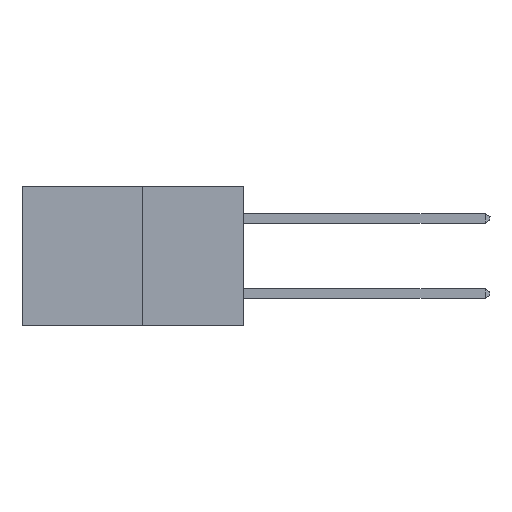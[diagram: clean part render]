
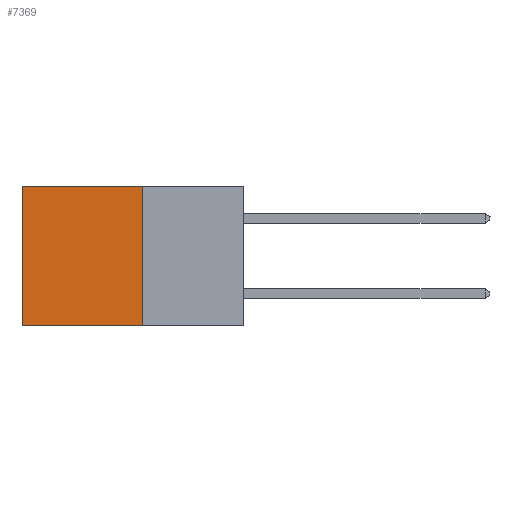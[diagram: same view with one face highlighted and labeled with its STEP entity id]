
A CAD part, left-side view. The second image highlights one B-rep face of the part: STEP entity #7369.
In plain terms, the highlighted planar face has unit normal (-1, 0, 0).
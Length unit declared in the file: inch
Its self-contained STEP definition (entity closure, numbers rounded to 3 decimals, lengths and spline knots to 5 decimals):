
#693 = AXIS2_PLACEMENT_3D ( 'NONE', #26904, #10281, #29672 ) ;
#1352 = VERTEX_POINT ( 'NONE', #14864 ) ;
#1359 = CARTESIAN_POINT ( 'NONE',  ( 0.277, 0.27, -0.37 ) ) ;
#3016 = VECTOR ( 'NONE', #18110, 39.37008 ) ;
#5978 = ORIENTED_EDGE ( 'NONE', *, *, #6654, .T. ) ;
#6654 = EDGE_CURVE ( 'NONE', #26735, #32204, #28831, .T. ) ;
#6737 = CARTESIAN_POINT ( 'NONE',  ( 0.277, 0.59, 0. ) ) ;
#6918 = ORIENTED_EDGE ( 'NONE', *, *, #29499, .F. ) ;
#7369 = ADVANCED_FACE ( 'NONE', ( #20980 ), #7477, .F. ) ;
#7477 = PLANE ( 'NONE',  #693 ) ;
#10281 = DIRECTION ( 'NONE',  ( 1., 0., 0. ) ) ;
#10402 = VECTOR ( 'NONE', #33155, 39.37008 ) ;
#11714 = EDGE_CURVE ( 'NONE', #1352, #35198, #17893, .T. ) ;
#12230 = CARTESIAN_POINT ( 'NONE',  ( 0.277, 0.59, -0.37 ) ) ;
#12426 = VECTOR ( 'NONE', #29361, 39.37008 ) ;
#12638 = DIRECTION ( 'NONE',  ( 0., 0., -1. ) ) ;
#14152 = LINE ( 'NONE', #31970, #12426 ) ;
#14864 = CARTESIAN_POINT ( 'NONE',  ( 0.277, 0.27, 0. ) ) ;
#17893 = LINE ( 'NONE', #1359, #3016 ) ;
#18110 = DIRECTION ( 'NONE',  ( 0., 0., -1. ) ) ;
#18461 = EDGE_CURVE ( 'NONE', #1352, #26735, #14152, .T. ) ;
#20570 = ORIENTED_EDGE ( 'NONE', *, *, #11714, .F. ) ;
#20980 = FACE_OUTER_BOUND ( 'NONE', #26748, .T. ) ;
#21452 = VECTOR ( 'NONE', #12638, 39.37008 ) ;
#26456 = CARTESIAN_POINT ( 'NONE',  ( 0.277, 0.59, -0.37 ) ) ;
#26735 = VERTEX_POINT ( 'NONE', #6737 ) ;
#26748 = EDGE_LOOP ( 'NONE', ( #5978, #6918, #20570, #31355 ) ) ;
#26904 = CARTESIAN_POINT ( 'NONE',  ( 0.277, 0.27, -0.37 ) ) ;
#28831 = LINE ( 'NONE', #26456, #21452 ) ;
#29361 = DIRECTION ( 'NONE',  ( 0., 1., 0. ) ) ;
#29499 = EDGE_CURVE ( 'NONE', #35198, #32204, #32457, .T. ) ;
#29672 = DIRECTION ( 'NONE',  ( 0., 0., -1. ) ) ;
#30450 = CARTESIAN_POINT ( 'NONE',  ( 0.277, 0.27, -0.37 ) ) ;
#31355 = ORIENTED_EDGE ( 'NONE', *, *, #18461, .T. ) ;
#31970 = CARTESIAN_POINT ( 'NONE',  ( 0.277, 0.27, 0. ) ) ;
#32204 = VERTEX_POINT ( 'NONE', #12230 ) ;
#32457 = LINE ( 'NONE', #30450, #10402 ) ;
#33155 = DIRECTION ( 'NONE',  ( 0., 1., 0. ) ) ;
#34549 = CARTESIAN_POINT ( 'NONE',  ( 0.277, 0.27, -0.37 ) ) ;
#35198 = VERTEX_POINT ( 'NONE', #34549 ) ;
